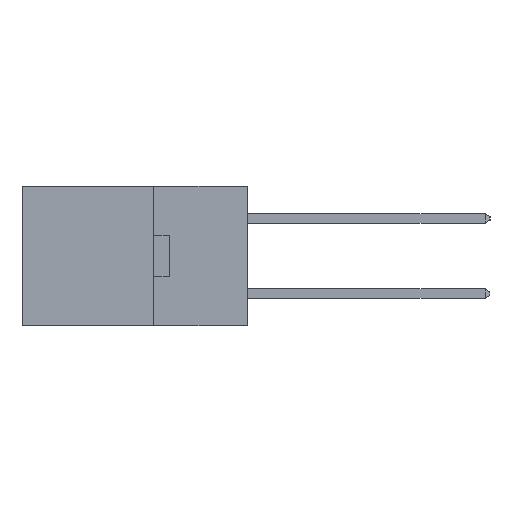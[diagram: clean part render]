
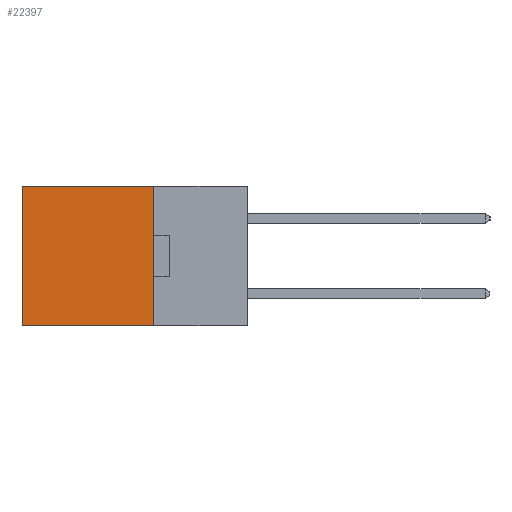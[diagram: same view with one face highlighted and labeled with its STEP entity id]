
A CAD part, left-side view. The second image highlights one B-rep face of the part: STEP entity #22397.
In plain terms, the highlighted planar face has unit normal (-1, 0, 0).
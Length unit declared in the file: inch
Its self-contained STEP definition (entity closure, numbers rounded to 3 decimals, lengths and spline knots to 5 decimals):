
#491 = VECTOR ( 'NONE', #13698, 39.37008 ) ;
#1059 = CARTESIAN_POINT ( 'NONE',  ( 0.2615, 0.25, -0.37 ) ) ;
#1352 = EDGE_LOOP ( 'NONE', ( #7355, #3322, #19665, #7854 ) ) ;
#1530 = AXIS2_PLACEMENT_3D ( 'NONE', #8741, #10882, #25764 ) ;
#1574 = DIRECTION ( 'NONE',  ( 0., 0., -1. ) ) ;
#1994 = FACE_OUTER_BOUND ( 'NONE', #1352, .T. ) ;
#2604 = VERTEX_POINT ( 'NONE', #4494 ) ;
#3322 = ORIENTED_EDGE ( 'NONE', *, *, #24475, .F. ) ;
#4494 = CARTESIAN_POINT ( 'NONE',  ( 0.2615, 0.6, 0. ) ) ;
#5032 = CARTESIAN_POINT ( 'NONE',  ( 0.2615, 0.25, -0.37 ) ) ;
#6528 = PLANE ( 'NONE',  #1530 ) ;
#7355 = ORIENTED_EDGE ( 'NONE', *, *, #14418, .T. ) ;
#7854 = ORIENTED_EDGE ( 'NONE', *, *, #9487, .T. ) ;
#8741 = CARTESIAN_POINT ( 'NONE',  ( 0.2615, 0.25, -0.37 ) ) ;
#9487 = EDGE_CURVE ( 'NONE', #22320, #2604, #22783, .T. ) ;
#10691 = LINE ( 'NONE', #5032, #491 ) ;
#10882 = DIRECTION ( 'NONE',  ( 1., 0., 0. ) ) ;
#11438 = VECTOR ( 'NONE', #15748, 39.37008 ) ;
#11539 = CARTESIAN_POINT ( 'NONE',  ( 0.2615, 0.25, -0.37 ) ) ;
#13698 = DIRECTION ( 'NONE',  ( 0., 0., -1. ) ) ;
#14418 = EDGE_CURVE ( 'NONE', #2604, #18196, #23762, .T. ) ;
#14439 = CARTESIAN_POINT ( 'NONE',  ( 0.2615, 0.6, -0.37 ) ) ;
#15318 = CARTESIAN_POINT ( 'NONE',  ( 0.2615, 0.6, -0.37 ) ) ;
#15748 = DIRECTION ( 'NONE',  ( 0., 1., 0. ) ) ;
#16043 = VECTOR ( 'NONE', #16163, 39.37008 ) ;
#16163 = DIRECTION ( 'NONE',  ( 0., 1., 0. ) ) ;
#17037 = CARTESIAN_POINT ( 'NONE',  ( 0.2615, 0.25, 0. ) ) ;
#17423 = VECTOR ( 'NONE', #1574, 39.37008 ) ;
#17870 = CARTESIAN_POINT ( 'NONE',  ( 0.2615, 0.25, 0. ) ) ;
#18196 = VERTEX_POINT ( 'NONE', #15318 ) ;
#18392 = EDGE_CURVE ( 'NONE', #22320, #22613, #10691, .T. ) ;
#19665 = ORIENTED_EDGE ( 'NONE', *, *, #18392, .F. ) ;
#22320 = VERTEX_POINT ( 'NONE', #17037 ) ;
#22397 = ADVANCED_FACE ( 'NONE', ( #1994 ), #6528, .F. ) ;
#22613 = VERTEX_POINT ( 'NONE', #11539 ) ;
#22783 = LINE ( 'NONE', #17870, #11438 ) ;
#23762 = LINE ( 'NONE', #14439, #17423 ) ;
#24475 = EDGE_CURVE ( 'NONE', #22613, #18196, #26656, .T. ) ;
#25764 = DIRECTION ( 'NONE',  ( 0., 0., -1. ) ) ;
#26656 = LINE ( 'NONE', #1059, #16043 ) ;
